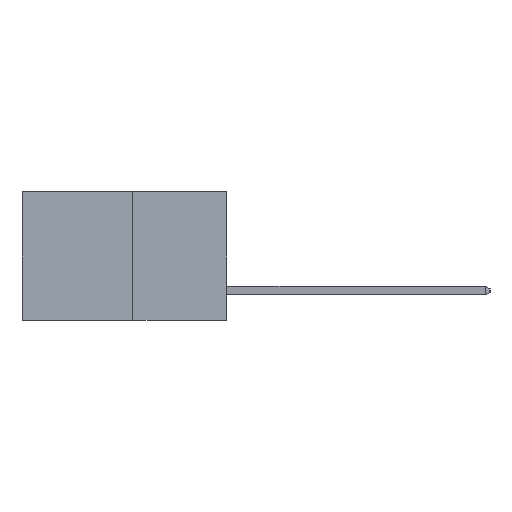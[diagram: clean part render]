
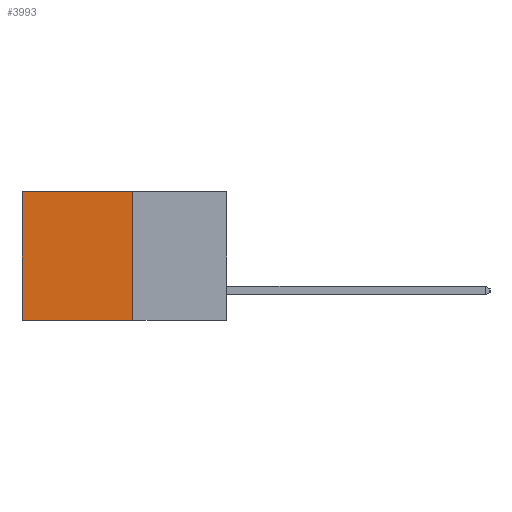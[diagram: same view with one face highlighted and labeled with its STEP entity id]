
A CAD part, left-side view. The second image highlights one B-rep face of the part: STEP entity #3993.
In plain terms, the highlighted planar face has unit normal (-1, 0, 0).
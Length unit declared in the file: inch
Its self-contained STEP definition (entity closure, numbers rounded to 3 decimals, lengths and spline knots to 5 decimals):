
#689 = DIRECTION ( 'NONE',  ( 0., 1., 0. ) ) ;
#939 = FACE_OUTER_BOUND ( 'NONE', #7096, .T. ) ;
#1102 = DIRECTION ( 'NONE',  ( 0., 0., -1. ) ) ;
#1242 = CARTESIAN_POINT ( 'NONE',  ( 0.277, 0.27, -0.37 ) ) ;
#1347 = LINE ( 'NONE', #5371, #3773 ) ;
#1610 = ORIENTED_EDGE ( 'NONE', *, *, #2040, .T. ) ;
#1821 = EDGE_CURVE ( 'NONE', #6938, #8021, #1842, .T. ) ;
#1842 = LINE ( 'NONE', #10025, #6863 ) ;
#1916 = DIRECTION ( 'NONE',  ( 0., 0., -1. ) ) ;
#1946 = DIRECTION ( 'NONE',  ( 1., 0., 0. ) ) ;
#2040 = EDGE_CURVE ( 'NONE', #5043, #7382, #1347, .T. ) ;
#2986 = EDGE_CURVE ( 'NONE', #5043, #6938, #4047, .T. ) ;
#3393 = AXIS2_PLACEMENT_3D ( 'NONE', #11419, #1946, #1916 ) ;
#3760 = CARTESIAN_POINT ( 'NONE',  ( 0.277, 0.59, -0.37 ) ) ;
#3773 = VECTOR ( 'NONE', #689, 39.37008 ) ;
#3791 = DIRECTION ( 'NONE',  ( 0., 0., -1. ) ) ;
#3993 = ADVANCED_FACE ( 'NONE', ( #939 ), #9558, .F. ) ;
#4047 = LINE ( 'NONE', #1242, #8929 ) ;
#5043 = VERTEX_POINT ( 'NONE', #9045 ) ;
#5123 = LINE ( 'NONE', #3760, #9881 ) ;
#5371 = CARTESIAN_POINT ( 'NONE',  ( 0.277, 0.27, 0. ) ) ;
#6328 = DIRECTION ( 'NONE',  ( 0., 1., 0. ) ) ;
#6863 = VECTOR ( 'NONE', #6328, 39.37008 ) ;
#6938 = VERTEX_POINT ( 'NONE', #11506 ) ;
#7096 = EDGE_LOOP ( 'NONE', ( #9992, #10830, #10147, #1610 ) ) ;
#7382 = VERTEX_POINT ( 'NONE', #8882 ) ;
#8021 = VERTEX_POINT ( 'NONE', #11144 ) ;
#8882 = CARTESIAN_POINT ( 'NONE',  ( 0.277, 0.59, 0. ) ) ;
#8929 = VECTOR ( 'NONE', #1102, 39.37008 ) ;
#9045 = CARTESIAN_POINT ( 'NONE',  ( 0.277, 0.27, 0. ) ) ;
#9345 = EDGE_CURVE ( 'NONE', #7382, #8021, #5123, .T. ) ;
#9558 = PLANE ( 'NONE',  #3393 ) ;
#9881 = VECTOR ( 'NONE', #3791, 39.37008 ) ;
#9992 = ORIENTED_EDGE ( 'NONE', *, *, #9345, .T. ) ;
#10025 = CARTESIAN_POINT ( 'NONE',  ( 0.277, 0.27, -0.37 ) ) ;
#10147 = ORIENTED_EDGE ( 'NONE', *, *, #2986, .F. ) ;
#10830 = ORIENTED_EDGE ( 'NONE', *, *, #1821, .F. ) ;
#11144 = CARTESIAN_POINT ( 'NONE',  ( 0.277, 0.59, -0.37 ) ) ;
#11419 = CARTESIAN_POINT ( 'NONE',  ( 0.277, 0.27, -0.37 ) ) ;
#11506 = CARTESIAN_POINT ( 'NONE',  ( 0.277, 0.27, -0.37 ) ) ;
